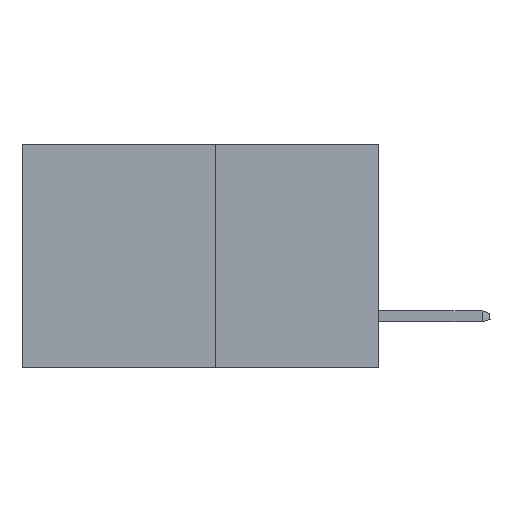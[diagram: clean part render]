
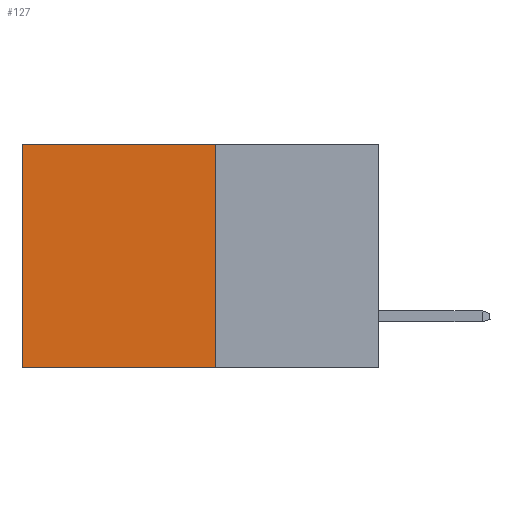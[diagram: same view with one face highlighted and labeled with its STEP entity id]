
A CAD part, left-side view. The second image highlights one B-rep face of the part: STEP entity #127.
In plain terms, the highlighted planar face has unit normal (-1, 0, 0).
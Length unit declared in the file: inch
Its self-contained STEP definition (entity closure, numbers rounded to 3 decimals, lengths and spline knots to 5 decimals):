
#127 = ADVANCED_FACE ( 'NONE', ( #16399 ), #19614, .F. ) ;
#815 = VECTOR ( 'NONE', #13294, 39.37008 ) ;
#2321 = VECTOR ( 'NONE', #4900, 39.37008 ) ;
#3353 = CARTESIAN_POINT ( 'NONE',  ( 0.277, 0.27, 0. ) ) ;
#4666 = AXIS2_PLACEMENT_3D ( 'NONE', #19814, #12849, #19669 ) ;
#4752 = ORIENTED_EDGE ( 'NONE', *, *, #17638, .F. ) ;
#4900 = DIRECTION ( 'NONE',  ( 0., 0., -1. ) ) ;
#4969 = CARTESIAN_POINT ( 'NONE',  ( 0.277, 0.59, -0.37 ) ) ;
#5644 = CARTESIAN_POINT ( 'NONE',  ( 0.277, 0.59, -0.37 ) ) ;
#6279 = CARTESIAN_POINT ( 'NONE',  ( 0.277, 0.27, -0.37 ) ) ;
#6349 = CARTESIAN_POINT ( 'NONE',  ( 0.277, 0.59, 0. ) ) ;
#6445 = LINE ( 'NONE', #4969, #2321 ) ;
#6690 = VERTEX_POINT ( 'NONE', #6349 ) ;
#6750 = EDGE_CURVE ( 'NONE', #6690, #20790, #6445, .T. ) ;
#6873 = LINE ( 'NONE', #6279, #7419 ) ;
#7419 = VECTOR ( 'NONE', #8016, 39.37008 ) ;
#8016 = DIRECTION ( 'NONE',  ( 0., 0., -1. ) ) ;
#8145 = CARTESIAN_POINT ( 'NONE',  ( 0.277, 0.27, 0. ) ) ;
#8442 = LINE ( 'NONE', #13557, #21477 ) ;
#10177 = DIRECTION ( 'NONE',  ( 0., 1., 0. ) ) ;
#11002 = ORIENTED_EDGE ( 'NONE', *, *, #21125, .T. ) ;
#11202 = VERTEX_POINT ( 'NONE', #3353 ) ;
#11793 = CARTESIAN_POINT ( 'NONE',  ( 0.277, 0.27, -0.37 ) ) ;
#12849 = DIRECTION ( 'NONE',  ( 1., 0., 0. ) ) ;
#13294 = DIRECTION ( 'NONE',  ( 0., 1., 0. ) ) ;
#13557 = CARTESIAN_POINT ( 'NONE',  ( 0.277, 0.27, -0.37 ) ) ;
#14255 = ORIENTED_EDGE ( 'NONE', *, *, #6750, .T. ) ;
#14285 = VERTEX_POINT ( 'NONE', #11793 ) ;
#14468 = EDGE_LOOP ( 'NONE', ( #14255, #16597, #4752, #11002 ) ) ;
#14680 = LINE ( 'NONE', #8145, #815 ) ;
#16399 = FACE_OUTER_BOUND ( 'NONE', #14468, .T. ) ;
#16597 = ORIENTED_EDGE ( 'NONE', *, *, #18471, .F. ) ;
#17638 = EDGE_CURVE ( 'NONE', #11202, #14285, #6873, .T. ) ;
#18471 = EDGE_CURVE ( 'NONE', #14285, #20790, #8442, .T. ) ;
#19614 = PLANE ( 'NONE',  #4666 ) ;
#19669 = DIRECTION ( 'NONE',  ( 0., 0., -1. ) ) ;
#19814 = CARTESIAN_POINT ( 'NONE',  ( 0.277, 0.27, -0.37 ) ) ;
#20790 = VERTEX_POINT ( 'NONE', #5644 ) ;
#21125 = EDGE_CURVE ( 'NONE', #11202, #6690, #14680, .T. ) ;
#21477 = VECTOR ( 'NONE', #10177, 39.37008 ) ;
